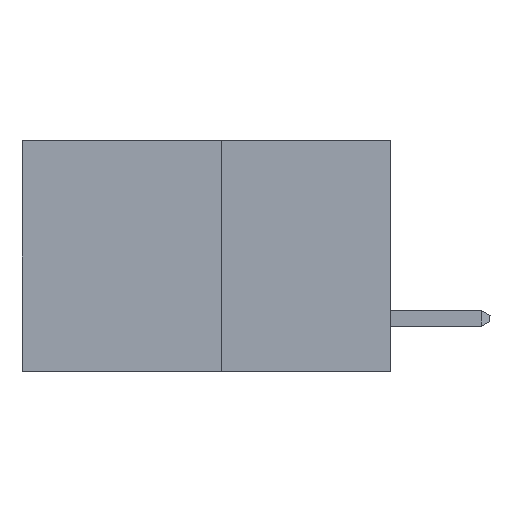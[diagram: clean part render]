
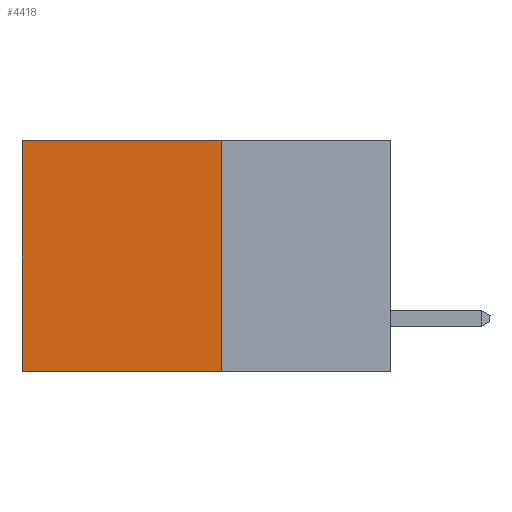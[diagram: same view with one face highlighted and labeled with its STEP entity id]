
A CAD part, left-side view. The second image highlights one B-rep face of the part: STEP entity #4418.
In plain terms, the highlighted planar face has unit normal (-1, 0, 0).
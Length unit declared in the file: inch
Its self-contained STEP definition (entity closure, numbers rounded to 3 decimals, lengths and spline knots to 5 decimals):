
#308 = EDGE_CURVE ( 'NONE', #1155, #5471, #3210, .T. ) ;
#406 = EDGE_CURVE ( 'NONE', #5471, #9050, #6694, .T. ) ;
#1155 = VERTEX_POINT ( 'NONE', #8307 ) ;
#1376 = CARTESIAN_POINT ( 'NONE',  ( 0.277, 0.27, -0.37 ) ) ;
#1437 = ORIENTED_EDGE ( 'NONE', *, *, #308, .T. ) ;
#1447 = DIRECTION ( 'NONE',  ( 0., 1., 0. ) ) ;
#1772 = FACE_OUTER_BOUND ( 'NONE', #3390, .T. ) ;
#2891 = VECTOR ( 'NONE', #1447, 39.37008 ) ;
#3210 = LINE ( 'NONE', #8667, #2891 ) ;
#3390 = EDGE_LOOP ( 'NONE', ( #10531, #10722, #11023, #1437 ) ) ;
#3980 = VECTOR ( 'NONE', #13128, 39.37008 ) ;
#4314 = AXIS2_PLACEMENT_3D ( 'NONE', #1376, #11516, #5453 ) ;
#4401 = PLANE ( 'NONE',  #4314 ) ;
#4418 = ADVANCED_FACE ( 'NONE', ( #1772 ), #4401, .F. ) ;
#5205 = CARTESIAN_POINT ( 'NONE',  ( 0.277, 0.59, -0.37 ) ) ;
#5453 = DIRECTION ( 'NONE',  ( 0., 0., -1. ) ) ;
#5471 = VERTEX_POINT ( 'NONE', #12821 ) ;
#6618 = CARTESIAN_POINT ( 'NONE',  ( 0.277, 0.27, -0.37 ) ) ;
#6694 = LINE ( 'NONE', #5205, #3980 ) ;
#7135 = DIRECTION ( 'NONE',  ( 0., 0., -1. ) ) ;
#7617 = DIRECTION ( 'NONE',  ( 0., 1., 0. ) ) ;
#7640 = LINE ( 'NONE', #12177, #10011 ) ;
#7806 = VERTEX_POINT ( 'NONE', #11469 ) ;
#8307 = CARTESIAN_POINT ( 'NONE',  ( 0.277, 0.27, 0. ) ) ;
#8667 = CARTESIAN_POINT ( 'NONE',  ( 0.277, 0.27, 0. ) ) ;
#8824 = EDGE_CURVE ( 'NONE', #1155, #7806, #7640, .T. ) ;
#9050 = VERTEX_POINT ( 'NONE', #10514 ) ;
#9523 = VECTOR ( 'NONE', #7617, 39.37008 ) ;
#9843 = LINE ( 'NONE', #6618, #9523 ) ;
#10011 = VECTOR ( 'NONE', #7135, 39.37008 ) ;
#10514 = CARTESIAN_POINT ( 'NONE',  ( 0.277, 0.59, -0.37 ) ) ;
#10531 = ORIENTED_EDGE ( 'NONE', *, *, #406, .T. ) ;
#10722 = ORIENTED_EDGE ( 'NONE', *, *, #11851, .F. ) ;
#11023 = ORIENTED_EDGE ( 'NONE', *, *, #8824, .F. ) ;
#11469 = CARTESIAN_POINT ( 'NONE',  ( 0.277, 0.27, -0.37 ) ) ;
#11516 = DIRECTION ( 'NONE',  ( 1., 0., 0. ) ) ;
#11851 = EDGE_CURVE ( 'NONE', #7806, #9050, #9843, .T. ) ;
#12177 = CARTESIAN_POINT ( 'NONE',  ( 0.277, 0.27, -0.37 ) ) ;
#12821 = CARTESIAN_POINT ( 'NONE',  ( 0.277, 0.59, 0. ) ) ;
#13128 = DIRECTION ( 'NONE',  ( 0., 0., -1. ) ) ;
